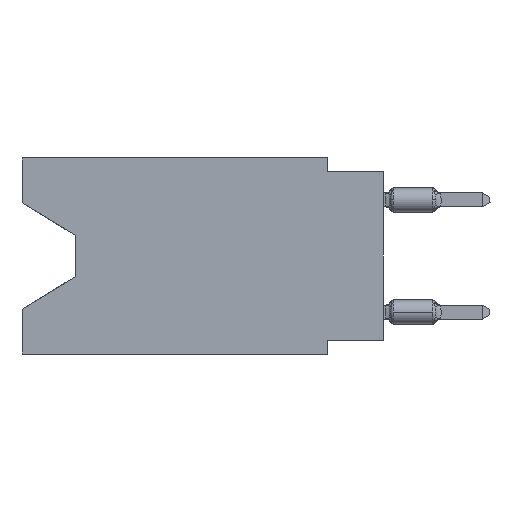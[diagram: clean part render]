
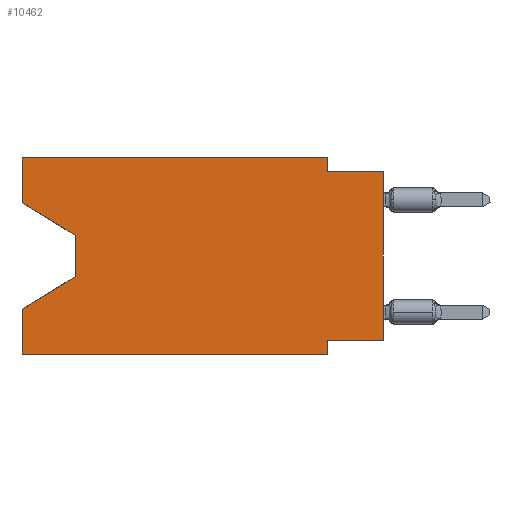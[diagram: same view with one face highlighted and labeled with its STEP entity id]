
A CAD part, left-side view. The second image highlights one B-rep face of the part: STEP entity #10462.
In plain terms, the highlighted planar face has unit normal (-1, 0, 0).
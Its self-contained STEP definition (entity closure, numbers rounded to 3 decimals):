
#3 = VECTOR ( 'NONE', #12616, 1000. ) ;
#152 = DIRECTION ( 'NONE',  ( 0., 0., -1. ) ) ;
#353 = ORIENTED_EDGE ( 'NONE', *, *, #7981, .T. ) ;
#771 = EDGE_CURVE ( 'NONE', #7523, #4974, #14913, .T. ) ;
#910 = VECTOR ( 'NONE', #12720, 1000. ) ;
#913 = DIRECTION ( 'NONE',  ( 0., -1., 0. ) ) ;
#967 = CARTESIAN_POINT ( 'NONE',  ( 0., 16.383, -2.038 ) ) ;
#1026 = ORIENTED_EDGE ( 'NONE', *, *, #1861, .T. ) ;
#1077 = DIRECTION ( 'NONE',  ( 1., 0., 0. ) ) ;
#1482 = ORIENTED_EDGE ( 'NONE', *, *, #18958, .T. ) ;
#1583 = EDGE_CURVE ( 'NONE', #8760, #6458, #10743, .T. ) ;
#1852 = ORIENTED_EDGE ( 'NONE', *, *, #1583, .F. ) ;
#1861 = EDGE_CURVE ( 'NONE', #4438, #14732, #11914, .T. ) ;
#2121 = DIRECTION ( 'NONE',  ( 0., 0., -1. ) ) ;
#2139 = CARTESIAN_POINT ( 'NONE',  ( 0., 16.383, 0. ) ) ;
#2157 = ORIENTED_EDGE ( 'NONE', *, *, #7979, .F. ) ;
#2462 = DIRECTION ( 'NONE',  ( 0., 0., 1. ) ) ;
#2540 = CARTESIAN_POINT ( 'NONE',  ( 0., 16.383, -6.852 ) ) ;
#2785 = VECTOR ( 'NONE', #15119, 1000. ) ;
#2848 = CARTESIAN_POINT ( 'NONE',  ( 0., 0., -0.635 ) ) ;
#2871 = CARTESIAN_POINT ( 'NONE',  ( 0., 16.383, 0. ) ) ;
#2933 = CARTESIAN_POINT ( 'NONE',  ( 0., 2.54, 0. ) ) ;
#3190 = EDGE_LOOP ( 'NONE', ( #19643, #1026, #18459, #12957, #1482, #8653, #10475, #353, #2157, #19856, #20767, #1852 ) ) ;
#3389 = VECTOR ( 'NONE', #152, 1000. ) ;
#3489 = CARTESIAN_POINT ( 'NONE',  ( 0., 16.383, 0. ) ) ;
#3744 = CARTESIAN_POINT ( 'NONE',  ( 0., 2.54, -8.89 ) ) ;
#4075 = VERTEX_POINT ( 'NONE', #17309 ) ;
#4330 = LINE ( 'NONE', #10991, #3 ) ;
#4344 = DIRECTION ( 'NONE',  ( 0., 0.855, -0.519 ) ) ;
#4438 = VERTEX_POINT ( 'NONE', #18783 ) ;
#4551 = FACE_OUTER_BOUND ( 'NONE', #3190, .T. ) ;
#4887 = LINE ( 'NONE', #8706, #2785 ) ;
#4974 = VERTEX_POINT ( 'NONE', #12736 ) ;
#5351 = DIRECTION ( 'NONE',  ( 0., 0., 1. ) ) ;
#5602 = VECTOR ( 'NONE', #4344, 1000. ) ;
#5786 = CARTESIAN_POINT ( 'NONE',  ( 0., 13.97, -5.385 ) ) ;
#5882 = VECTOR ( 'NONE', #913, 1000. ) ;
#6193 = DIRECTION ( 'NONE',  ( 0., -0.855, -0.519 ) ) ;
#6413 = CARTESIAN_POINT ( 'NONE',  ( 0., 16.383, 0. ) ) ;
#6458 = VERTEX_POINT ( 'NONE', #3489 ) ;
#7523 = VERTEX_POINT ( 'NONE', #19620 ) ;
#7524 = VERTEX_POINT ( 'NONE', #2848 ) ;
#7845 = LINE ( 'NONE', #5786, #5602 ) ;
#7882 = CARTESIAN_POINT ( 'NONE',  ( 0., 13.97, -5.385 ) ) ;
#7979 = EDGE_CURVE ( 'NONE', #4974, #7524, #4330, .T. ) ;
#7981 = EDGE_CURVE ( 'NONE', #4075, #7524, #9476, .T. ) ;
#7993 = LINE ( 'NONE', #9835, #19162 ) ;
#8286 = VECTOR ( 'NONE', #2121, 1000. ) ;
#8653 = ORIENTED_EDGE ( 'NONE', *, *, #9821, .F. ) ;
#8706 = CARTESIAN_POINT ( 'NONE',  ( 0., 16.383, -8.89 ) ) ;
#8751 = CARTESIAN_POINT ( 'NONE',  ( 0., 2.54, -8.255 ) ) ;
#8760 = VERTEX_POINT ( 'NONE', #20180 ) ;
#8857 = EDGE_CURVE ( 'NONE', #11082, #9984, #14724, .T. ) ;
#8903 = CARTESIAN_POINT ( 'NONE',  ( 0., 2.54, -8.89 ) ) ;
#9055 = EDGE_CURVE ( 'NONE', #8760, #4438, #14455, .T. ) ;
#9476 = LINE ( 'NONE', #11213, #10792 ) ;
#9821 = EDGE_CURVE ( 'NONE', #11409, #13092, #13752, .T. ) ;
#9835 = CARTESIAN_POINT ( 'NONE',  ( 0., 0., -8.255 ) ) ;
#9984 = VERTEX_POINT ( 'NONE', #2540 ) ;
#10462 = ADVANCED_FACE ( 'NONE', ( #4551 ), #16210, .F. ) ;
#10475 = ORIENTED_EDGE ( 'NONE', *, *, #16824, .F. ) ;
#10743 = LINE ( 'NONE', #2139, #11028 ) ;
#10792 = VECTOR ( 'NONE', #21015, 1000. ) ;
#10929 = CARTESIAN_POINT ( 'NONE',  ( 0., 16.383, -8.89 ) ) ;
#10991 = CARTESIAN_POINT ( 'NONE',  ( 0., 0., -0.635 ) ) ;
#11028 = VECTOR ( 'NONE', #2462, 1000. ) ;
#11045 = VECTOR ( 'NONE', #6193, 1000. ) ;
#11082 = VERTEX_POINT ( 'NONE', #10929 ) ;
#11114 = EDGE_CURVE ( 'NONE', #6458, #7523, #19105, .T. ) ;
#11204 = DIRECTION ( 'NONE',  ( 0., 0., -1. ) ) ;
#11213 = CARTESIAN_POINT ( 'NONE',  ( 0., 0., 0. ) ) ;
#11409 = VERTEX_POINT ( 'NONE', #8751 ) ;
#11776 = AXIS2_PLACEMENT_3D ( 'NONE', #6413, #1077, #11204 ) ;
#11914 = LINE ( 'NONE', #18350, #3389 ) ;
#12616 = DIRECTION ( 'NONE',  ( 0., -1., 0. ) ) ;
#12720 = DIRECTION ( 'NONE',  ( 0., 0., -1. ) ) ;
#12736 = CARTESIAN_POINT ( 'NONE',  ( 0., 2.54, -0.635 ) ) ;
#12957 = ORIENTED_EDGE ( 'NONE', *, *, #8857, .F. ) ;
#13092 = VERTEX_POINT ( 'NONE', #8903 ) ;
#13752 = LINE ( 'NONE', #3744, #8286 ) ;
#14455 = LINE ( 'NONE', #967, #11045 ) ;
#14724 = LINE ( 'NONE', #15371, #19057 ) ;
#14729 = DIRECTION ( 'NONE',  ( 0., 1., 0. ) ) ;
#14732 = VERTEX_POINT ( 'NONE', #7882 ) ;
#14913 = LINE ( 'NONE', #2933, #910 ) ;
#15119 = DIRECTION ( 'NONE',  ( 0., -1., 0. ) ) ;
#15371 = CARTESIAN_POINT ( 'NONE',  ( 0., 16.383, 0. ) ) ;
#16210 = PLANE ( 'NONE',  #11776 ) ;
#16824 = EDGE_CURVE ( 'NONE', #4075, #11409, #7993, .T. ) ;
#17038 = EDGE_CURVE ( 'NONE', #14732, #9984, #7845, .T. ) ;
#17309 = CARTESIAN_POINT ( 'NONE',  ( 0., 0., -8.255 ) ) ;
#18350 = CARTESIAN_POINT ( 'NONE',  ( 0., 13.97, -3.505 ) ) ;
#18459 = ORIENTED_EDGE ( 'NONE', *, *, #17038, .T. ) ;
#18783 = CARTESIAN_POINT ( 'NONE',  ( 0., 13.97, -3.505 ) ) ;
#18958 = EDGE_CURVE ( 'NONE', #11082, #13092, #4887, .T. ) ;
#19057 = VECTOR ( 'NONE', #5351, 1000. ) ;
#19105 = LINE ( 'NONE', #2871, #5882 ) ;
#19162 = VECTOR ( 'NONE', #14729, 1000. ) ;
#19620 = CARTESIAN_POINT ( 'NONE',  ( 0., 2.54, 0. ) ) ;
#19643 = ORIENTED_EDGE ( 'NONE', *, *, #9055, .T. ) ;
#19856 = ORIENTED_EDGE ( 'NONE', *, *, #771, .F. ) ;
#20180 = CARTESIAN_POINT ( 'NONE',  ( 0., 16.383, -2.038 ) ) ;
#20767 = ORIENTED_EDGE ( 'NONE', *, *, #11114, .F. ) ;
#21015 = DIRECTION ( 'NONE',  ( 0., 0., 1. ) ) ;
